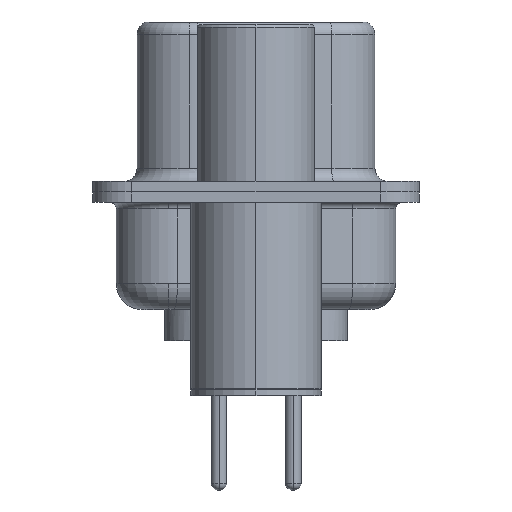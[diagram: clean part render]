
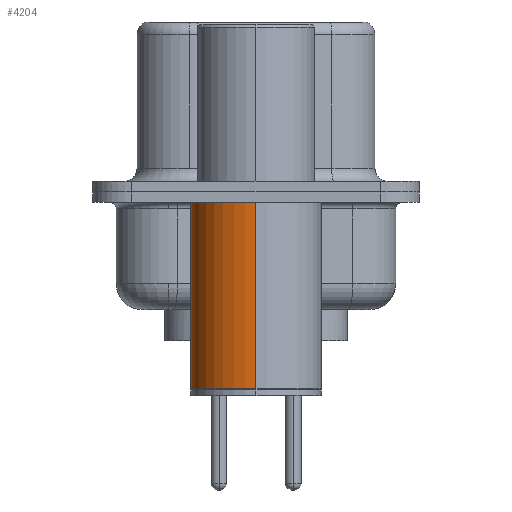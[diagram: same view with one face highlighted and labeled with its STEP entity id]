
A CAD part, left-side view. The second image highlights one B-rep face of the part: STEP entity #4204.
In plain terms, the highlighted cylindrical face has radius 2.5 mm (diameter 5 mm), a partial arc.
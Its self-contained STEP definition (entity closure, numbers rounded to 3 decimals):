
#78 = AXIS2_PLACEMENT_3D ( 'NONE', #12186, #2205, #10679 ) ;
#368 = DIRECTION ( 'NONE',  ( 0., 0., 1. ) ) ;
#627 = VERTEX_POINT ( 'NONE', #2710 ) ;
#763 = EDGE_CURVE ( 'NONE', #627, #2068, #12876, .T. ) ;
#1091 = EDGE_LOOP ( 'NONE', ( #6785, #4848, #17815, #14484 ) ) ;
#2068 = VERTEX_POINT ( 'NONE', #17480 ) ;
#2205 = DIRECTION ( 'NONE',  ( 0., 0., 1. ) ) ;
#2710 = CARTESIAN_POINT ( 'NONE',  ( 2.5, 0., -7.525 ) ) ;
#4018 = DIRECTION ( 'NONE',  ( 0., 0., 1. ) ) ;
#4204 = ADVANCED_FACE ( 'NONE', ( #11609 ), #17534, .T. ) ;
#4341 = DIRECTION ( 'NONE',  ( 0., 0., 1. ) ) ;
#4401 = CARTESIAN_POINT ( 'NONE',  ( -2.5, 0., 0.581 ) ) ;
#4848 = ORIENTED_EDGE ( 'NONE', *, *, #7001, .T. ) ;
#6124 = VERTEX_POINT ( 'NONE', #13078 ) ;
#6785 = ORIENTED_EDGE ( 'NONE', *, *, #16244, .T. ) ;
#7001 = EDGE_CURVE ( 'NONE', #8573, #6124, #15793, .T. ) ;
#7127 = AXIS2_PLACEMENT_3D ( 'NONE', #14819, #368, #9113 ) ;
#7160 = DIRECTION ( 'NONE',  ( 1., 0., 0. ) ) ;
#8573 = VERTEX_POINT ( 'NONE', #14357 ) ;
#9113 = DIRECTION ( 'NONE',  ( 1., 0., 0. ) ) ;
#9683 = AXIS2_PLACEMENT_3D ( 'NONE', #15991, #14379, #7160 ) ;
#10091 = CIRCLE ( 'NONE', #78, 2.5 ) ;
#10679 = DIRECTION ( 'NONE',  ( 1., 0., 0. ) ) ;
#11609 = FACE_OUTER_BOUND ( 'NONE', #1091, .T. ) ;
#12186 = CARTESIAN_POINT ( 'NONE',  ( 0., 0., -7.525 ) ) ;
#12876 = LINE ( 'NONE', #18695, #13782 ) ;
#13078 = CARTESIAN_POINT ( 'NONE',  ( -2.5, 0., -0.4 ) ) ;
#13291 = EDGE_CURVE ( 'NONE', #2068, #6124, #15021, .T. ) ;
#13782 = VECTOR ( 'NONE', #4341, 1000. ) ;
#14357 = CARTESIAN_POINT ( 'NONE',  ( -2.5, 0., -7.525 ) ) ;
#14379 = DIRECTION ( 'NONE',  ( 0., 0., 1. ) ) ;
#14484 = ORIENTED_EDGE ( 'NONE', *, *, #763, .F. ) ;
#14819 = CARTESIAN_POINT ( 'NONE',  ( 0., 0., -0.4 ) ) ;
#15021 = CIRCLE ( 'NONE', #7127, 2.5 ) ;
#15793 = LINE ( 'NONE', #4401, #18274 ) ;
#15991 = CARTESIAN_POINT ( 'NONE',  ( 0., 0., 0.581 ) ) ;
#16244 = EDGE_CURVE ( 'NONE', #627, #8573, #10091, .T. ) ;
#17480 = CARTESIAN_POINT ( 'NONE',  ( 2.5, 0., -0.4 ) ) ;
#17534 = CYLINDRICAL_SURFACE ( 'NONE', #9683, 2.5 ) ;
#17815 = ORIENTED_EDGE ( 'NONE', *, *, #13291, .F. ) ;
#18274 = VECTOR ( 'NONE', #4018, 1000. ) ;
#18695 = CARTESIAN_POINT ( 'NONE',  ( 2.5, 0., 0.581 ) ) ;
